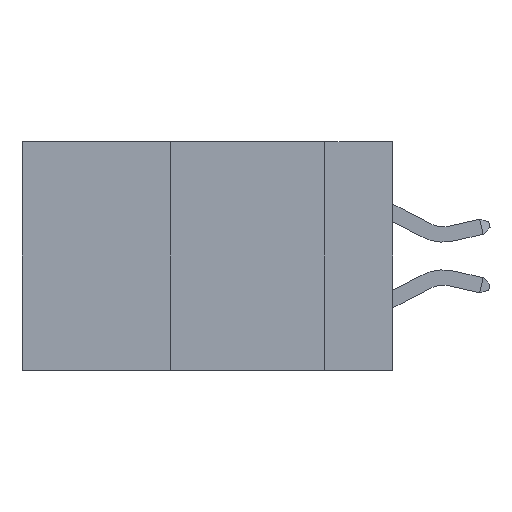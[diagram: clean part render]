
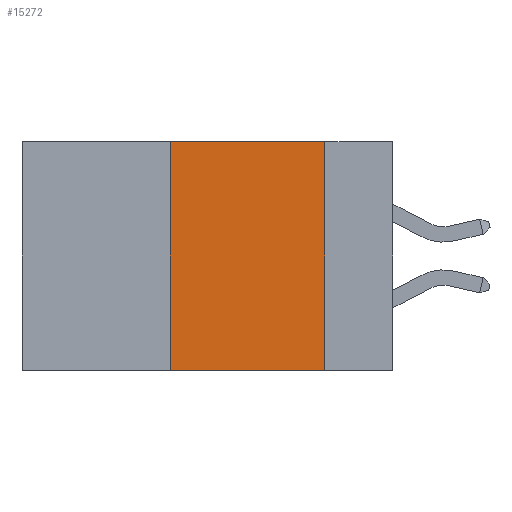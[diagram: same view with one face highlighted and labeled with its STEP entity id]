
A CAD part, left-side view. The second image highlights one B-rep face of the part: STEP entity #15272.
In plain terms, the highlighted planar face has unit normal (-1, 0, 0).
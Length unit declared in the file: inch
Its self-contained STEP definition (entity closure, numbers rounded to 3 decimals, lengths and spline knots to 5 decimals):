
#121 = CARTESIAN_POINT ( 'NONE',  ( 0., 0.11, 0. ) ) ;
#819 = CARTESIAN_POINT ( 'NONE',  ( 0., 0.36, 0. ) ) ;
#1285 = VERTEX_POINT ( 'NONE', #16755 ) ;
#1759 = CARTESIAN_POINT ( 'NONE',  ( 0., 0.11, -0.37 ) ) ;
#2074 = LINE ( 'NONE', #121, #15281 ) ;
#2632 = DIRECTION ( 'NONE',  ( 0., -1., 0. ) ) ;
#2809 = LINE ( 'NONE', #6661, #6017 ) ;
#3359 = EDGE_LOOP ( 'NONE', ( #5373, #15800, #13837, #15218 ) ) ;
#4155 = EDGE_CURVE ( 'NONE', #12337, #14469, #2074, .T. ) ;
#4713 = PLANE ( 'NONE',  #15544 ) ;
#5093 = EDGE_CURVE ( 'NONE', #1285, #8010, #11400, .T. ) ;
#5373 = ORIENTED_EDGE ( 'NONE', *, *, #4155, .F. ) ;
#5431 = VECTOR ( 'NONE', #8272, 39.37008 ) ;
#5863 = LINE ( 'NONE', #6939, #5431 ) ;
#6017 = VECTOR ( 'NONE', #2632, 39.37008 ) ;
#6661 = CARTESIAN_POINT ( 'NONE',  ( 0., 0.6, 0. ) ) ;
#6939 = CARTESIAN_POINT ( 'NONE',  ( 0., 0.6, -0.37 ) ) ;
#7129 = VECTOR ( 'NONE', #15366, 39.37008 ) ;
#7423 = DIRECTION ( 'NONE',  ( 1., 0., 0. ) ) ;
#8010 = VERTEX_POINT ( 'NONE', #12428 ) ;
#8272 = DIRECTION ( 'NONE',  ( 0., -1., 0. ) ) ;
#8980 = EDGE_CURVE ( 'NONE', #1285, #14469, #5863, .T. ) ;
#9568 = DIRECTION ( 'NONE',  ( 0., 0., -1. ) ) ;
#11400 = LINE ( 'NONE', #819, #7129 ) ;
#12171 = FACE_OUTER_BOUND ( 'NONE', #3359, .T. ) ;
#12337 = VERTEX_POINT ( 'NONE', #14689 ) ;
#12428 = CARTESIAN_POINT ( 'NONE',  ( 0., 0.36, 0. ) ) ;
#13837 = ORIENTED_EDGE ( 'NONE', *, *, #5093, .F. ) ;
#14469 = VERTEX_POINT ( 'NONE', #1759 ) ;
#14689 = CARTESIAN_POINT ( 'NONE',  ( 0., 0.11, 0. ) ) ;
#15175 = CARTESIAN_POINT ( 'NONE',  ( 0., 0.6, 0. ) ) ;
#15218 = ORIENTED_EDGE ( 'NONE', *, *, #8980, .T. ) ;
#15272 = ADVANCED_FACE ( 'NONE', ( #12171 ), #4713, .F. ) ;
#15281 = VECTOR ( 'NONE', #9568, 39.37008 ) ;
#15366 = DIRECTION ( 'NONE',  ( 0., 0., 1. ) ) ;
#15544 = AXIS2_PLACEMENT_3D ( 'NONE', #15175, #7423, #16450 ) ;
#15800 = ORIENTED_EDGE ( 'NONE', *, *, #16721, .F. ) ;
#16450 = DIRECTION ( 'NONE',  ( 0., 0., -1. ) ) ;
#16721 = EDGE_CURVE ( 'NONE', #8010, #12337, #2809, .T. ) ;
#16755 = CARTESIAN_POINT ( 'NONE',  ( 0., 0.36, -0.37 ) ) ;
